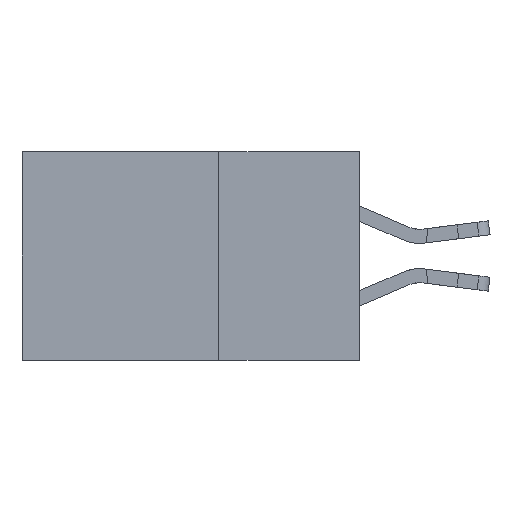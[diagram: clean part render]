
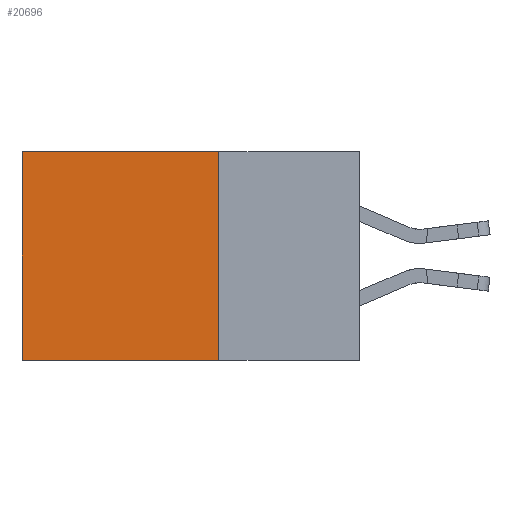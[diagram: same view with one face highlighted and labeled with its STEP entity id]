
A CAD part, left-side view. The second image highlights one B-rep face of the part: STEP entity #20696.
In plain terms, the highlighted planar face has unit normal (-1, 0, 0).
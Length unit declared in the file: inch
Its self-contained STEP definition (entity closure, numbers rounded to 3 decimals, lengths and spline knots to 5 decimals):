
#951 = VECTOR ( 'NONE', #2920, 39.37008 ) ;
#1022 = DIRECTION ( 'NONE',  ( 1., 0., 0. ) ) ;
#1127 = EDGE_CURVE ( 'NONE', #5631, #9756, #21090, .T. ) ;
#1632 = CARTESIAN_POINT ( 'NONE',  ( 0.2875, 0.6, -0.37 ) ) ;
#2254 = CARTESIAN_POINT ( 'NONE',  ( 0.2875, 0.6, 0. ) ) ;
#2569 = AXIS2_PLACEMENT_3D ( 'NONE', #18993, #1022, #9013 ) ;
#2920 = DIRECTION ( 'NONE',  ( 0., 1., 0. ) ) ;
#2959 = VECTOR ( 'NONE', #24288, 39.37008 ) ;
#2976 = PLANE ( 'NONE',  #2569 ) ;
#5631 = VERTEX_POINT ( 'NONE', #22355 ) ;
#5865 = ORIENTED_EDGE ( 'NONE', *, *, #11728, .F. ) ;
#6278 = VECTOR ( 'NONE', #19237, 39.37008 ) ;
#6672 = CARTESIAN_POINT ( 'NONE',  ( 0.2875, 0.6, 0. ) ) ;
#6838 = LINE ( 'NONE', #23375, #951 ) ;
#7187 = CARTESIAN_POINT ( 'NONE',  ( 0.2875, 0.25, -0.37 ) ) ;
#8536 = VERTEX_POINT ( 'NONE', #7187 ) ;
#8844 = ORIENTED_EDGE ( 'NONE', *, *, #1127, .T. ) ;
#8901 = DIRECTION ( 'NONE',  ( 0., 0., -1. ) ) ;
#9013 = DIRECTION ( 'NONE',  ( 0., 0., -1. ) ) ;
#9207 = EDGE_LOOP ( 'NONE', ( #15917, #11840, #5865, #8844 ) ) ;
#9756 = VERTEX_POINT ( 'NONE', #6672 ) ;
#10986 = CARTESIAN_POINT ( 'NONE',  ( 0.2875, 0.25, 0. ) ) ;
#11728 = EDGE_CURVE ( 'NONE', #5631, #8536, #25039, .T. ) ;
#11840 = ORIENTED_EDGE ( 'NONE', *, *, #22715, .F. ) ;
#15490 = VERTEX_POINT ( 'NONE', #1632 ) ;
#15917 = ORIENTED_EDGE ( 'NONE', *, *, #20144, .T. ) ;
#17141 = FACE_OUTER_BOUND ( 'NONE', #9207, .T. ) ;
#18993 = CARTESIAN_POINT ( 'NONE',  ( 0.2875, 0.25, 0. ) ) ;
#19237 = DIRECTION ( 'NONE',  ( 0., 1., 0. ) ) ;
#20144 = EDGE_CURVE ( 'NONE', #9756, #15490, #20228, .T. ) ;
#20228 = LINE ( 'NONE', #2254, #2959 ) ;
#20696 = ADVANCED_FACE ( 'NONE', ( #17141 ), #2976, .F. ) ;
#21090 = LINE ( 'NONE', #10986, #6278 ) ;
#21523 = VECTOR ( 'NONE', #8901, 39.37008 ) ;
#22355 = CARTESIAN_POINT ( 'NONE',  ( 0.2875, 0.25, 0. ) ) ;
#22715 = EDGE_CURVE ( 'NONE', #8536, #15490, #6838, .T. ) ;
#23050 = CARTESIAN_POINT ( 'NONE',  ( 0.2875, 0.25, 0. ) ) ;
#23375 = CARTESIAN_POINT ( 'NONE',  ( 0.2875, 0.25, -0.37 ) ) ;
#24288 = DIRECTION ( 'NONE',  ( 0., 0., -1. ) ) ;
#25039 = LINE ( 'NONE', #23050, #21523 ) ;
